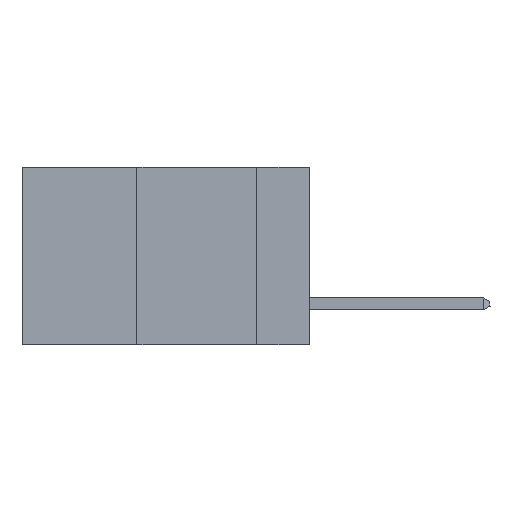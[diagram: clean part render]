
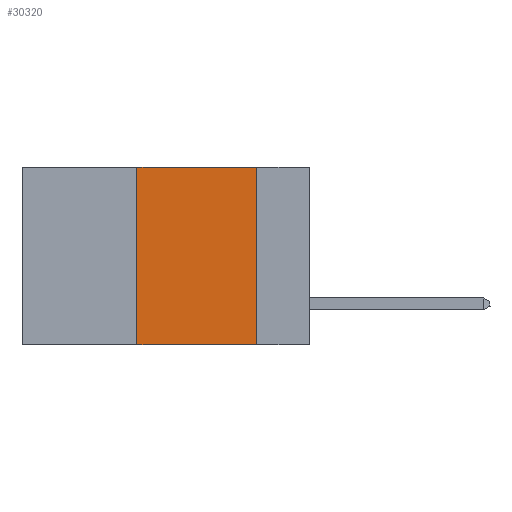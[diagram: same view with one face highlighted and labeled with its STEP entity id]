
A CAD part, left-side view. The second image highlights one B-rep face of the part: STEP entity #30320.
In plain terms, the highlighted planar face has unit normal (-1, 0, 0).
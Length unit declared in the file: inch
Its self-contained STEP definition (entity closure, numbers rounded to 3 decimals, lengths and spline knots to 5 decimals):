
#1500 = ORIENTED_EDGE ( 'NONE', *, *, #30056, .F. ) ;
#1700 = CARTESIAN_POINT ( 'NONE',  ( 0., 0.11, -0.37 ) ) ;
#1782 = VECTOR ( 'NONE', #35433, 39.37008 ) ;
#2049 = CARTESIAN_POINT ( 'NONE',  ( 0., 0.11, 0. ) ) ;
#3144 = CARTESIAN_POINT ( 'NONE',  ( 0., 0.11, 0. ) ) ;
#4365 = EDGE_CURVE ( 'NONE', #33153, #6840, #35874, .T. ) ;
#6840 = VERTEX_POINT ( 'NONE', #3144 ) ;
#8729 = ORIENTED_EDGE ( 'NONE', *, *, #23969, .T. ) ;
#9691 = VECTOR ( 'NONE', #10460, 39.37008 ) ;
#10460 = DIRECTION ( 'NONE',  ( 0., -1., 0. ) ) ;
#12452 = DIRECTION ( 'NONE',  ( 0., 0., 1. ) ) ;
#12815 = LINE ( 'NONE', #2049, #1782 ) ;
#15435 = LINE ( 'NONE', #34652, #22991 ) ;
#16212 = VERTEX_POINT ( 'NONE', #36642 ) ;
#20983 = CARTESIAN_POINT ( 'NONE',  ( 0., 0.6, 0. ) ) ;
#22806 = EDGE_LOOP ( 'NONE', ( #25318, #25924, #1500, #8729 ) ) ;
#22991 = VECTOR ( 'NONE', #12452, 39.37008 ) ;
#23245 = CARTESIAN_POINT ( 'NONE',  ( 0., 0.36, 0. ) ) ;
#23969 = EDGE_CURVE ( 'NONE', #16212, #43238, #46111, .T. ) ;
#25080 = DIRECTION ( 'NONE',  ( 0., -1., 0. ) ) ;
#25318 = ORIENTED_EDGE ( 'NONE', *, *, #41542, .F. ) ;
#25439 = CARTESIAN_POINT ( 'NONE',  ( 0., 0.6, 0. ) ) ;
#25924 = ORIENTED_EDGE ( 'NONE', *, *, #4365, .F. ) ;
#28452 = FACE_OUTER_BOUND ( 'NONE', #22806, .T. ) ;
#30056 = EDGE_CURVE ( 'NONE', #16212, #33153, #15435, .T. ) ;
#30320 = ADVANCED_FACE ( 'NONE', ( #28452 ), #47408, .F. ) ;
#32881 = DIRECTION ( 'NONE',  ( 1., 0., 0. ) ) ;
#33153 = VERTEX_POINT ( 'NONE', #23245 ) ;
#34652 = CARTESIAN_POINT ( 'NONE',  ( 0., 0.36, 0. ) ) ;
#35433 = DIRECTION ( 'NONE',  ( 0., 0., -1. ) ) ;
#35874 = LINE ( 'NONE', #20983, #43308 ) ;
#36642 = CARTESIAN_POINT ( 'NONE',  ( 0., 0.36, -0.37 ) ) ;
#39749 = CARTESIAN_POINT ( 'NONE',  ( 0., 0.6, -0.37 ) ) ;
#41542 = EDGE_CURVE ( 'NONE', #6840, #43238, #12815, .T. ) ;
#43238 = VERTEX_POINT ( 'NONE', #1700 ) ;
#43308 = VECTOR ( 'NONE', #25080, 39.37008 ) ;
#43899 = DIRECTION ( 'NONE',  ( 0., 0., -1. ) ) ;
#46111 = LINE ( 'NONE', #39749, #9691 ) ;
#46963 = AXIS2_PLACEMENT_3D ( 'NONE', #25439, #32881, #43899 ) ;
#47408 = PLANE ( 'NONE',  #46963 ) ;
